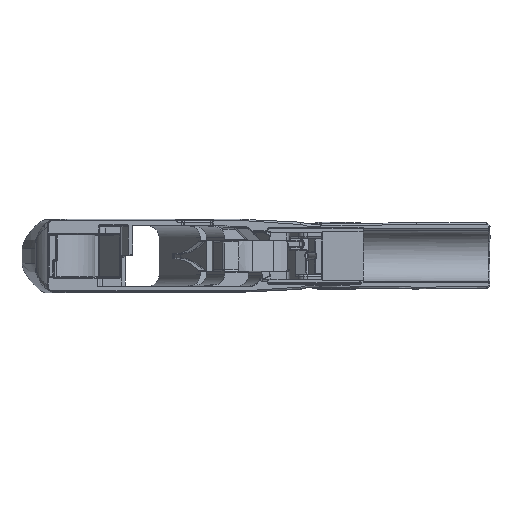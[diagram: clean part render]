
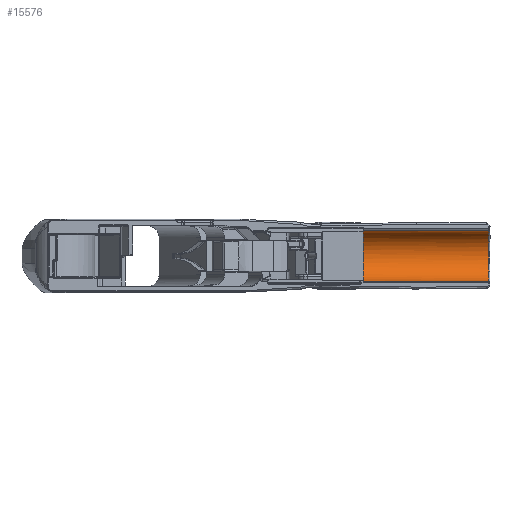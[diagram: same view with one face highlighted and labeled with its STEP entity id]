
A CAD part, top view. The second image highlights one B-rep face of the part: STEP entity #15576.
In plain terms, the highlighted cylindrical face has radius 8.75 mm (diameter 17.5 mm), a partial arc.
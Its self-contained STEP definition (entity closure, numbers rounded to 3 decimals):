
#1099=LINE('',#38808,#1753);
#1190=LINE('',#42183,#1844);
#1753=VECTOR('',#19133,1000.);
#1844=VECTOR('',#19552,1000.);
#2287=CIRCLE('',#16607,8.75);
#2292=CIRCLE('',#16614,8.75);
#2358=CIRCLE('',#16769,8.75);
#2359=CIRCLE('',#16773,8.75);
#2662=CYLINDRICAL_SURFACE('',#16772,8.75);
#6668=ORIENTED_EDGE('',*,*,#9655,.F.);
#6669=ORIENTED_EDGE('',*,*,#9656,.F.);
#6670=ORIENTED_EDGE('',*,*,#9323,.T.);
#6671=ORIENTED_EDGE('',*,*,#9318,.T.);
#6672=ORIENTED_EDGE('',*,*,#9314,.F.);
#6673=ORIENTED_EDGE('',*,*,#9647,.F.);
#9314=EDGE_CURVE('',#11103,#11104,#2287,.T.);
#9318=EDGE_CURVE('',#11106,#11104,#1099,.T.);
#9323=EDGE_CURVE('',#11108,#11106,#2292,.T.);
#9647=EDGE_CURVE('',#11299,#11103,#2358,.T.);
#9655=EDGE_CURVE('',#11303,#11299,#2359,.T.);
#9656=EDGE_CURVE('',#11108,#11303,#1190,.T.);
#11103=VERTEX_POINT('',#38800);
#11104=VERTEX_POINT('',#38802);
#11106=VERTEX_POINT('',#38809);
#11108=VERTEX_POINT('',#38814);
#11299=VERTEX_POINT('',#42144);
#11303=VERTEX_POINT('',#42182);
#13454=EDGE_LOOP('',(#6668,#6669,#6670,#6671,#6672,#6673));
#14432=FACE_BOUND('',#13454,.T.);
#15576=ADVANCED_FACE('',(#14432),#2662,.F.);
#16607=AXIS2_PLACEMENT_3D('',#38801,#19125,#19126);
#16614=AXIS2_PLACEMENT_3D('',#38818,#19143,#19144);
#16769=AXIS2_PLACEMENT_3D('',#42143,#19537,#19538);
#16772=AXIS2_PLACEMENT_3D('',#42180,#19548,#19549);
#16773=AXIS2_PLACEMENT_3D('',#42181,#19550,#19551);
#19125=DIRECTION('',(1.,0.,0.));
#19126=DIRECTION('',(0.,0.,1.));
#19133=DIRECTION('',(-1.,0.,0.));
#19143=DIRECTION('',(1.,0.,0.));
#19144=DIRECTION('',(0.,0.,-1.));
#19537=DIRECTION('',(1.,0.,0.));
#19538=DIRECTION('',(0.,0.,1.));
#19548=DIRECTION('',(-1.,0.,0.));
#19549=DIRECTION('',(0.,-1.,0.));
#19550=DIRECTION('',(1.,0.,0.));
#19551=DIRECTION('',(0.,0.,1.));
#19552=DIRECTION('',(-1.,0.,0.));
#38800=CARTESIAN_POINT('',(32.829,8.375,20.716));
#38801=CARTESIAN_POINT('',(32.829,0.,23.25));
#38802=CARTESIAN_POINT('',(32.829,8.75,23.25));
#38808=CARTESIAN_POINT('',(76.25,8.75,23.25));
#38809=CARTESIAN_POINT('',(75.75,8.75,23.25));
#38814=CARTESIAN_POINT('',(75.75,-8.75,23.25));
#38818=CARTESIAN_POINT('',(75.75,0.,23.25));
#42143=CARTESIAN_POINT('',(32.829,0.,23.25));
#42144=CARTESIAN_POINT('',(32.829,-8.5,21.173));
#42180=CARTESIAN_POINT('',(76.25,0.,23.25));
#42181=CARTESIAN_POINT('',(32.829,0.,23.25));
#42182=CARTESIAN_POINT('',(32.829,-8.75,23.25));
#42183=CARTESIAN_POINT('',(76.25,-8.75,23.25));
